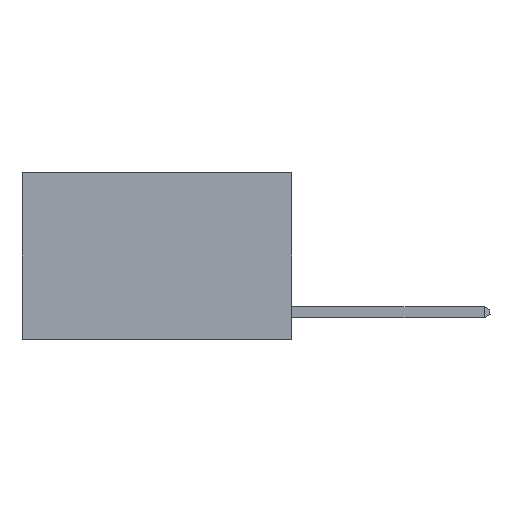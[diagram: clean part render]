
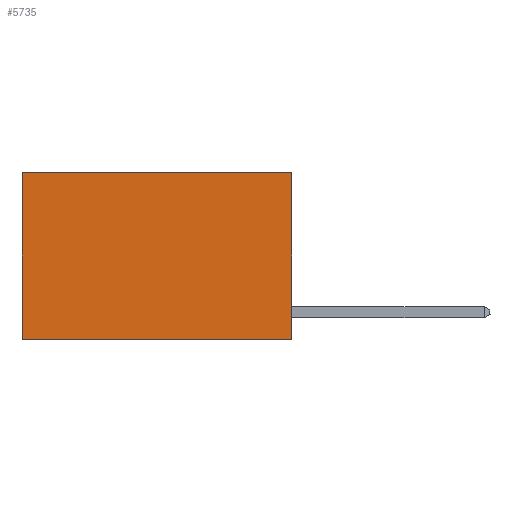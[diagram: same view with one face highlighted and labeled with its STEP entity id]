
A CAD part, left-side view. The second image highlights one B-rep face of the part: STEP entity #5735.
In plain terms, the highlighted planar face has unit normal (-1, 0, 0).
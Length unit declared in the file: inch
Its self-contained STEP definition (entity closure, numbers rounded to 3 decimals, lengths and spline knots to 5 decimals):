
#1411 = VERTEX_POINT ( 'NONE', #9107 ) ;
#1617 = DIRECTION ( 'NONE',  ( 0., 0., -1. ) ) ;
#2445 = EDGE_CURVE ( 'NONE', #4118, #5798, #2987, .T. ) ;
#2987 = LINE ( 'NONE', #23003, #22204 ) ;
#3470 = DIRECTION ( 'NONE',  ( 1., 0., 0. ) ) ;
#3547 = DIRECTION ( 'NONE',  ( 0., 1., 0. ) ) ;
#3562 = AXIS2_PLACEMENT_3D ( 'NONE', #18779, #3470, #1617 ) ;
#3648 = ORIENTED_EDGE ( 'NONE', *, *, #2445, .T. ) ;
#3771 = CARTESIAN_POINT ( 'NONE',  ( 0.2625, 0.6, -0.37 ) ) ;
#4118 = VERTEX_POINT ( 'NONE', #9800 ) ;
#5508 = CARTESIAN_POINT ( 'NONE',  ( 0.2625, 0.6, 0. ) ) ;
#5735 = ADVANCED_FACE ( 'NONE', ( #21196 ), #14486, .F. ) ;
#5798 = VERTEX_POINT ( 'NONE', #22912 ) ;
#5942 = EDGE_CURVE ( 'NONE', #1411, #9697, #8899, .T. ) ;
#7035 = EDGE_CURVE ( 'NONE', #5798, #9697, #7802, .T. ) ;
#7616 = EDGE_CURVE ( 'NONE', #4118, #1411, #17849, .T. ) ;
#7802 = LINE ( 'NONE', #5508, #18228 ) ;
#8899 = LINE ( 'NONE', #23769, #16818 ) ;
#9107 = CARTESIAN_POINT ( 'NONE',  ( 0.2625, 0., -0.37 ) ) ;
#9117 = VECTOR ( 'NONE', #16133, 39.37008 ) ;
#9697 = VERTEX_POINT ( 'NONE', #3771 ) ;
#9800 = CARTESIAN_POINT ( 'NONE',  ( 0.2625, 0., 0. ) ) ;
#12231 = ORIENTED_EDGE ( 'NONE', *, *, #7035, .T. ) ;
#13188 = DIRECTION ( 'NONE',  ( 0., 1., 0. ) ) ;
#14486 = PLANE ( 'NONE',  #3562 ) ;
#14490 = ORIENTED_EDGE ( 'NONE', *, *, #7616, .F. ) ;
#16112 = DIRECTION ( 'NONE',  ( 0., 0., -1. ) ) ;
#16133 = DIRECTION ( 'NONE',  ( 0., 0., -1. ) ) ;
#16818 = VECTOR ( 'NONE', #13188, 39.37008 ) ;
#17849 = LINE ( 'NONE', #24554, #9117 ) ;
#18228 = VECTOR ( 'NONE', #16112, 39.37008 ) ;
#18779 = CARTESIAN_POINT ( 'NONE',  ( 0.2625, 0., 0. ) ) ;
#21196 = FACE_OUTER_BOUND ( 'NONE', #23407, .T. ) ;
#22204 = VECTOR ( 'NONE', #3547, 39.37008 ) ;
#22912 = CARTESIAN_POINT ( 'NONE',  ( 0.2625, 0.6, 0. ) ) ;
#23003 = CARTESIAN_POINT ( 'NONE',  ( 0.2625, 0., 0. ) ) ;
#23407 = EDGE_LOOP ( 'NONE', ( #12231, #26479, #14490, #3648 ) ) ;
#23769 = CARTESIAN_POINT ( 'NONE',  ( 0.2625, 0., -0.37 ) ) ;
#24554 = CARTESIAN_POINT ( 'NONE',  ( 0.2625, 0., 0. ) ) ;
#26479 = ORIENTED_EDGE ( 'NONE', *, *, #5942, .F. ) ;
